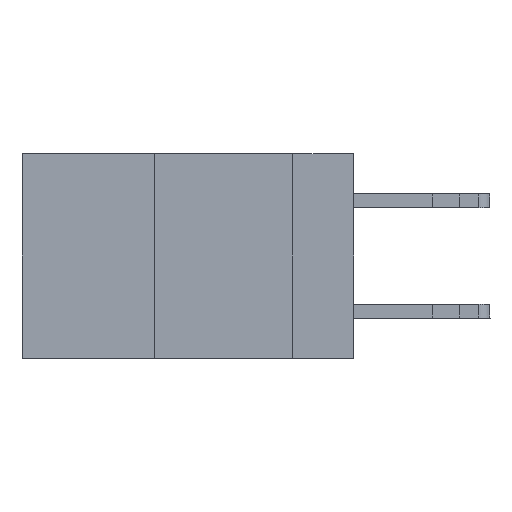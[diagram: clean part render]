
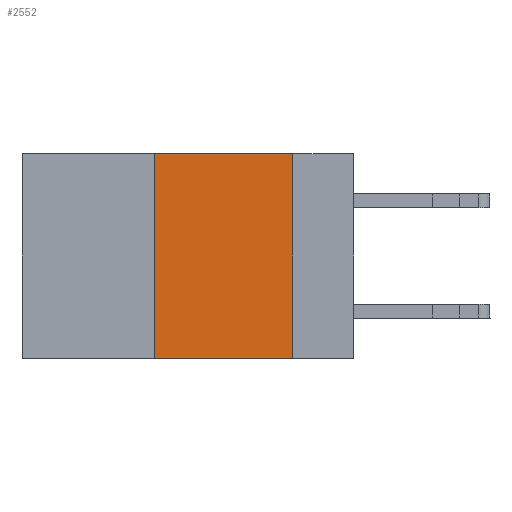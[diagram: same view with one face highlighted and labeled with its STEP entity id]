
A CAD part, left-side view. The second image highlights one B-rep face of the part: STEP entity #2552.
In plain terms, the highlighted planar face has unit normal (-1, 0, 0).
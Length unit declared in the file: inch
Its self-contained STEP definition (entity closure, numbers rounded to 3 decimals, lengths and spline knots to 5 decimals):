
#465 = ORIENTED_EDGE ( 'NONE', *, *, #6133, .F. ) ;
#1160 = DIRECTION ( 'NONE',  ( 0., -1., 0. ) ) ;
#1641 = DIRECTION ( 'NONE',  ( 0., 0., -1. ) ) ;
#2552 = ADVANCED_FACE ( 'NONE', ( #6639 ), #5777, .F. ) ;
#3427 = VERTEX_POINT ( 'NONE', #14687 ) ;
#4345 = CARTESIAN_POINT ( 'NONE',  ( 0., 0.36, 0. ) ) ;
#4880 = CARTESIAN_POINT ( 'NONE',  ( 0., 0.11, -0.37 ) ) ;
#5448 = LINE ( 'NONE', #22472, #19167 ) ;
#5692 = ORIENTED_EDGE ( 'NONE', *, *, #22883, .T. ) ;
#5777 = PLANE ( 'NONE',  #14331 ) ;
#6133 = EDGE_CURVE ( 'NONE', #11709, #14439, #6892, .T. ) ;
#6639 = FACE_OUTER_BOUND ( 'NONE', #7414, .T. ) ;
#6892 = LINE ( 'NONE', #6954, #14748 ) ;
#6954 = CARTESIAN_POINT ( 'NONE',  ( 0., 0.36, 0. ) ) ;
#7157 = VECTOR ( 'NONE', #22481, 39.37008 ) ;
#7233 = EDGE_CURVE ( 'NONE', #14439, #3427, #5448, .T. ) ;
#7414 = EDGE_LOOP ( 'NONE', ( #12976, #17729, #465, #5692 ) ) ;
#7521 = VECTOR ( 'NONE', #1641, 39.37008 ) ;
#7973 = VERTEX_POINT ( 'NONE', #4880 ) ;
#8617 = CARTESIAN_POINT ( 'NONE',  ( 0., 0.11, 0. ) ) ;
#9317 = DIRECTION ( 'NONE',  ( 0., 0., -1. ) ) ;
#11709 = VERTEX_POINT ( 'NONE', #14685 ) ;
#12279 = DIRECTION ( 'NONE',  ( 0., 0., 1. ) ) ;
#12976 = ORIENTED_EDGE ( 'NONE', *, *, #16179, .F. ) ;
#14331 = AXIS2_PLACEMENT_3D ( 'NONE', #19989, #20065, #9317 ) ;
#14439 = VERTEX_POINT ( 'NONE', #4345 ) ;
#14685 = CARTESIAN_POINT ( 'NONE',  ( 0., 0.36, -0.37 ) ) ;
#14687 = CARTESIAN_POINT ( 'NONE',  ( 0., 0.11, 0. ) ) ;
#14748 = VECTOR ( 'NONE', #12279, 39.37008 ) ;
#16179 = EDGE_CURVE ( 'NONE', #3427, #7973, #17065, .T. ) ;
#16703 = LINE ( 'NONE', #20684, #7157 ) ;
#17065 = LINE ( 'NONE', #8617, #7521 ) ;
#17729 = ORIENTED_EDGE ( 'NONE', *, *, #7233, .F. ) ;
#19167 = VECTOR ( 'NONE', #1160, 39.37008 ) ;
#19989 = CARTESIAN_POINT ( 'NONE',  ( 0., 0.6, 0. ) ) ;
#20065 = DIRECTION ( 'NONE',  ( 1., 0., 0. ) ) ;
#20684 = CARTESIAN_POINT ( 'NONE',  ( 0., 0.6, -0.37 ) ) ;
#22472 = CARTESIAN_POINT ( 'NONE',  ( 0., 0.6, 0. ) ) ;
#22481 = DIRECTION ( 'NONE',  ( 0., -1., 0. ) ) ;
#22883 = EDGE_CURVE ( 'NONE', #11709, #7973, #16703, .T. ) ;
